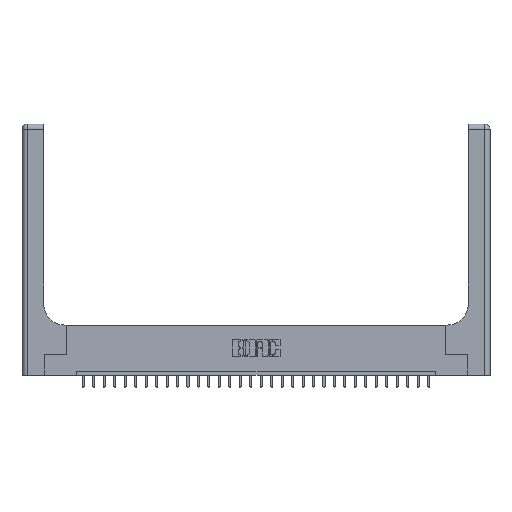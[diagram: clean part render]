
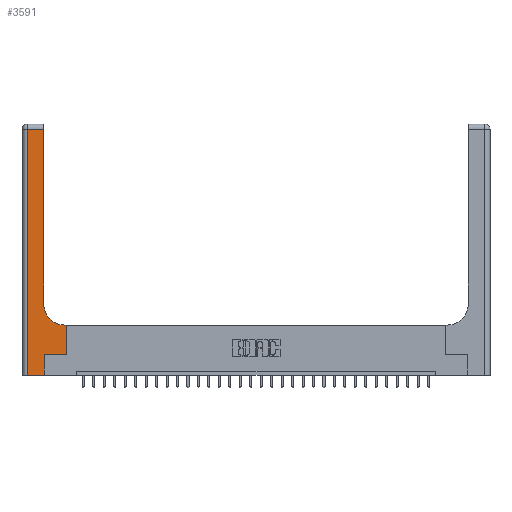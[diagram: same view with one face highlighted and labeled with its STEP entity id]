
A CAD part, top view. The second image highlights one B-rep face of the part: STEP entity #3591.
In plain terms, the highlighted planar face has unit normal (0, 0, 1).
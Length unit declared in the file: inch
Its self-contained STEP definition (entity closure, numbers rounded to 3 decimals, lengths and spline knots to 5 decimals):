
#101 = LINE ( 'NONE', #12905, #18232 ) ;
#594 = CARTESIAN_POINT ( 'NONE',  ( 0.265, 0.25, 0.37 ) ) ;
#674 = ORIENTED_EDGE ( 'NONE', *, *, #11940, .T. ) ;
#1056 = LINE ( 'NONE', #22583, #22855 ) ;
#1381 = CARTESIAN_POINT ( 'NONE',  ( 0.51, 0.85, 0.37 ) ) ;
#1452 = CARTESIAN_POINT ( 'NONE',  ( 0.265, 0.25, 0.37 ) ) ;
#1746 = CIRCLE ( 'NONE', #5345, 0.25 ) ;
#3163 = DIRECTION ( 'NONE',  ( 1., 0., 0. ) ) ;
#3172 = DIRECTION ( 'NONE',  ( -1., 0., 0. ) ) ;
#3268 = EDGE_CURVE ( 'NONE', #27638, #14249, #101, .T. ) ;
#3591 = ADVANCED_FACE ( 'NONE', ( #27100 ), #16139, .F. ) ;
#3659 = ORIENTED_EDGE ( 'NONE', *, *, #4847, .T. ) ;
#3733 = ORIENTED_EDGE ( 'NONE', *, *, #20084, .T. ) ;
#3853 = VERTEX_POINT ( 'NONE', #594 ) ;
#4618 = VERTEX_POINT ( 'NONE', #18090 ) ;
#4847 = EDGE_CURVE ( 'NONE', #12401, #22417, #6231, .T. ) ;
#5079 = VECTOR ( 'NONE', #16378, 39.37008 ) ;
#5345 = AXIS2_PLACEMENT_3D ( 'NONE', #1381, #14461, #23056 ) ;
#5565 = CARTESIAN_POINT ( 'NONE',  ( 0.26, 0.85, 0.37 ) ) ;
#5670 = EDGE_CURVE ( 'NONE', #16223, #18468, #19653, .T. ) ;
#5851 = CARTESIAN_POINT ( 'NONE',  ( 0.06, 2.94, 0.37 ) ) ;
#6231 = LINE ( 'NONE', #6788, #24105 ) ;
#6788 = CARTESIAN_POINT ( 'NONE',  ( 0.26, 3., 0.37 ) ) ;
#7508 = VECTOR ( 'NONE', #27753, 39.37008 ) ;
#7760 = VERTEX_POINT ( 'NONE', #9448 ) ;
#8762 = DIRECTION ( 'NONE',  ( 0., 1., 0. ) ) ;
#9092 = CARTESIAN_POINT ( 'NONE',  ( 0.06, 3., 0.37 ) ) ;
#9448 = CARTESIAN_POINT ( 'NONE',  ( 0.265, 0., 0.37 ) ) ;
#9493 = ORIENTED_EDGE ( 'NONE', *, *, #3268, .T. ) ;
#11940 = EDGE_CURVE ( 'NONE', #14249, #12401, #1746, .T. ) ;
#12159 = LINE ( 'NONE', #22705, #5079 ) ;
#12401 = VERTEX_POINT ( 'NONE', #5565 ) ;
#12497 = DIRECTION ( 'NONE',  ( -1., 0., 0. ) ) ;
#12905 = CARTESIAN_POINT ( 'NONE',  ( 0.26, 0.6, 0.37 ) ) ;
#13680 = EDGE_CURVE ( 'NONE', #4618, #27638, #21455, .T. ) ;
#13907 = EDGE_CURVE ( 'NONE', #7760, #3853, #12159, .T. ) ;
#14249 = VERTEX_POINT ( 'NONE', #20172 ) ;
#14461 = DIRECTION ( 'NONE',  ( 0., 0., -1. ) ) ;
#14757 = VECTOR ( 'NONE', #27004, 39.37008 ) ;
#15546 = DIRECTION ( 'NONE',  ( 0., -1., 0. ) ) ;
#16139 = PLANE ( 'NONE',  #24948 ) ;
#16223 = VERTEX_POINT ( 'NONE', #5851 ) ;
#16378 = DIRECTION ( 'NONE',  ( 0., 1., 0. ) ) ;
#16738 = ORIENTED_EDGE ( 'NONE', *, *, #24052, .T. ) ;
#17201 = VECTOR ( 'NONE', #25800, 39.37008 ) ;
#17246 = CARTESIAN_POINT ( 'NONE',  ( 0.528, 0.25, 0.37 ) ) ;
#18019 = LINE ( 'NONE', #24477, #14757 ) ;
#18090 = CARTESIAN_POINT ( 'NONE',  ( 0.528, 0.25, 0.37 ) ) ;
#18232 = VECTOR ( 'NONE', #12497, 39.37008 ) ;
#18468 = VERTEX_POINT ( 'NONE', #23641 ) ;
#18523 = CARTESIAN_POINT ( 'NONE',  ( 0., 3., 0.37 ) ) ;
#19034 = LINE ( 'NONE', #1452, #7508 ) ;
#19323 = ORIENTED_EDGE ( 'NONE', *, *, #13680, .T. ) ;
#19653 = LINE ( 'NONE', #9092, #25072 ) ;
#19759 = ORIENTED_EDGE ( 'NONE', *, *, #21986, .T. ) ;
#20084 = EDGE_CURVE ( 'NONE', #3853, #4618, #19034, .T. ) ;
#20172 = CARTESIAN_POINT ( 'NONE',  ( 0.51, 0.6, 0.37 ) ) ;
#21266 = CARTESIAN_POINT ( 'NONE',  ( 0.528, 0.6, 0.37 ) ) ;
#21455 = LINE ( 'NONE', #17246, #17201 ) ;
#21986 = EDGE_CURVE ( 'NONE', #22417, #16223, #18019, .T. ) ;
#22417 = VERTEX_POINT ( 'NONE', #22604 ) ;
#22476 = DIRECTION ( 'NONE',  ( 0., 0., -1. ) ) ;
#22583 = CARTESIAN_POINT ( 'NONE',  ( 0., 0., 0.37 ) ) ;
#22604 = CARTESIAN_POINT ( 'NONE',  ( 0.26, 2.94, 0.37 ) ) ;
#22705 = CARTESIAN_POINT ( 'NONE',  ( 0.265, 0., 0.37 ) ) ;
#22855 = VECTOR ( 'NONE', #3163, 39.37008 ) ;
#23056 = DIRECTION ( 'NONE',  ( 1., 0., 0. ) ) ;
#23641 = CARTESIAN_POINT ( 'NONE',  ( 0.06, 0., 0.37 ) ) ;
#24052 = EDGE_CURVE ( 'NONE', #18468, #7760, #1056, .T. ) ;
#24105 = VECTOR ( 'NONE', #8762, 39.37008 ) ;
#24477 = CARTESIAN_POINT ( 'NONE',  ( 0., 2.94, 0.37 ) ) ;
#24948 = AXIS2_PLACEMENT_3D ( 'NONE', #18523, #22476, #3172 ) ;
#25072 = VECTOR ( 'NONE', #15546, 39.37008 ) ;
#25800 = DIRECTION ( 'NONE',  ( 0., 1., 0. ) ) ;
#26103 = ORIENTED_EDGE ( 'NONE', *, *, #5670, .T. ) ;
#27004 = DIRECTION ( 'NONE',  ( -1., 0., 0. ) ) ;
#27084 = ORIENTED_EDGE ( 'NONE', *, *, #13907, .T. ) ;
#27100 = FACE_OUTER_BOUND ( 'NONE', #27626, .T. ) ;
#27626 = EDGE_LOOP ( 'NONE', ( #3659, #19759, #26103, #16738, #27084, #3733, #19323, #9493, #674 ) ) ;
#27638 = VERTEX_POINT ( 'NONE', #21266 ) ;
#27753 = DIRECTION ( 'NONE',  ( 1., 0., 0. ) ) ;
